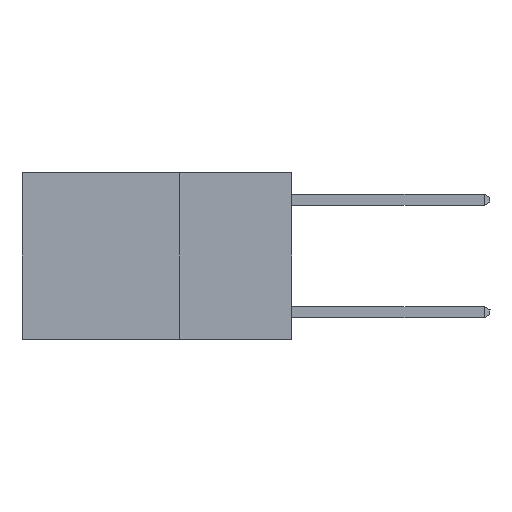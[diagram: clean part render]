
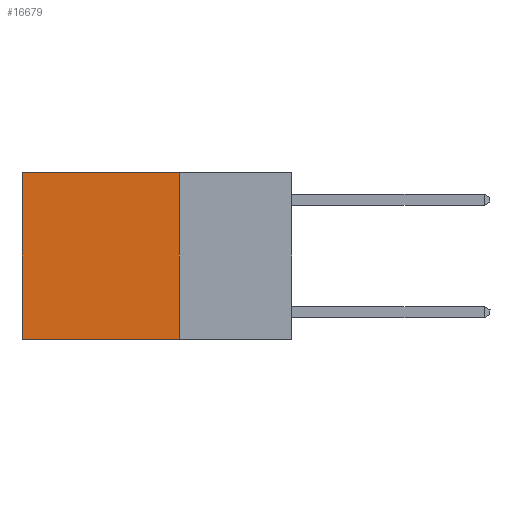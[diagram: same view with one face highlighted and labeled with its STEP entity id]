
A CAD part, left-side view. The second image highlights one B-rep face of the part: STEP entity #16679.
In plain terms, the highlighted planar face has unit normal (-1, 0, 0).
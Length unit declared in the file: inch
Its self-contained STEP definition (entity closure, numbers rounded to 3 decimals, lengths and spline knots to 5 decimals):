
#222 = CARTESIAN_POINT ( 'NONE',  ( 0.2625, 0.25, 0. ) ) ;
#860 = CARTESIAN_POINT ( 'NONE',  ( 0.2625, 0.25, 0. ) ) ;
#1506 = CARTESIAN_POINT ( 'NONE',  ( 0.2625, 0.6, 0. ) ) ;
#2236 = LINE ( 'NONE', #18372, #5424 ) ;
#2383 = LINE ( 'NONE', #222, #14092 ) ;
#3108 = CARTESIAN_POINT ( 'NONE',  ( 0.2625, 0.25, 0. ) ) ;
#4030 = DIRECTION ( 'NONE',  ( 1., 0., 0. ) ) ;
#5424 = VECTOR ( 'NONE', #6482, 39.37008 ) ;
#5570 = PLANE ( 'NONE',  #10364 ) ;
#6015 = VERTEX_POINT ( 'NONE', #1506 ) ;
#6020 = VERTEX_POINT ( 'NONE', #3108 ) ;
#6482 = DIRECTION ( 'NONE',  ( 0., 0., -1. ) ) ;
#6549 = FACE_OUTER_BOUND ( 'NONE', #18621, .T. ) ;
#7729 = CARTESIAN_POINT ( 'NONE',  ( 0.2625, 0.25, -0.37 ) ) ;
#8410 = CARTESIAN_POINT ( 'NONE',  ( 0.2625, 0.25, -0.37 ) ) ;
#8705 = ORIENTED_EDGE ( 'NONE', *, *, #12681, .F. ) ;
#9502 = LINE ( 'NONE', #18176, #16923 ) ;
#9677 = EDGE_CURVE ( 'NONE', #13480, #13389, #10246, .T. ) ;
#10246 = LINE ( 'NONE', #7729, #13732 ) ;
#10364 = AXIS2_PLACEMENT_3D ( 'NONE', #860, #4030, #14680 ) ;
#12575 = ORIENTED_EDGE ( 'NONE', *, *, #15184, .T. ) ;
#12681 = EDGE_CURVE ( 'NONE', #6020, #13480, #2383, .T. ) ;
#13389 = VERTEX_POINT ( 'NONE', #18614 ) ;
#13480 = VERTEX_POINT ( 'NONE', #8410 ) ;
#13732 = VECTOR ( 'NONE', #16646, 39.37008 ) ;
#13754 = ORIENTED_EDGE ( 'NONE', *, *, #9677, .F. ) ;
#14092 = VECTOR ( 'NONE', #18503, 39.37008 ) ;
#14680 = DIRECTION ( 'NONE',  ( 0., 0., -1. ) ) ;
#14690 = EDGE_CURVE ( 'NONE', #6015, #13389, #2236, .T. ) ;
#15184 = EDGE_CURVE ( 'NONE', #6020, #6015, #9502, .T. ) ;
#15694 = ORIENTED_EDGE ( 'NONE', *, *, #14690, .T. ) ;
#16646 = DIRECTION ( 'NONE',  ( 0., 1., 0. ) ) ;
#16675 = DIRECTION ( 'NONE',  ( 0., 1., 0. ) ) ;
#16679 = ADVANCED_FACE ( 'NONE', ( #6549 ), #5570, .F. ) ;
#16923 = VECTOR ( 'NONE', #16675, 39.37008 ) ;
#18176 = CARTESIAN_POINT ( 'NONE',  ( 0.2625, 0.25, 0. ) ) ;
#18372 = CARTESIAN_POINT ( 'NONE',  ( 0.2625, 0.6, 0. ) ) ;
#18503 = DIRECTION ( 'NONE',  ( 0., 0., -1. ) ) ;
#18614 = CARTESIAN_POINT ( 'NONE',  ( 0.2625, 0.6, -0.37 ) ) ;
#18621 = EDGE_LOOP ( 'NONE', ( #15694, #13754, #8705, #12575 ) ) ;
